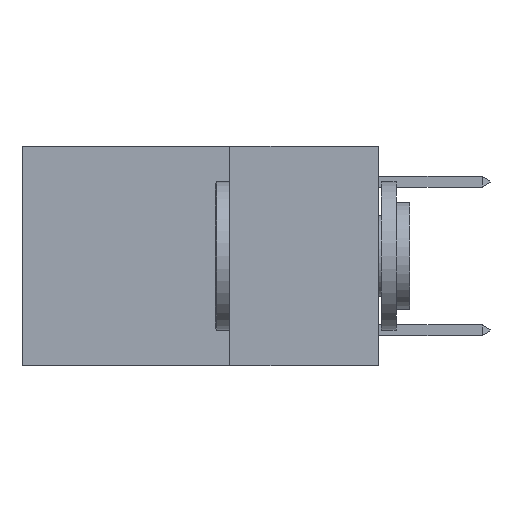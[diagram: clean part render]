
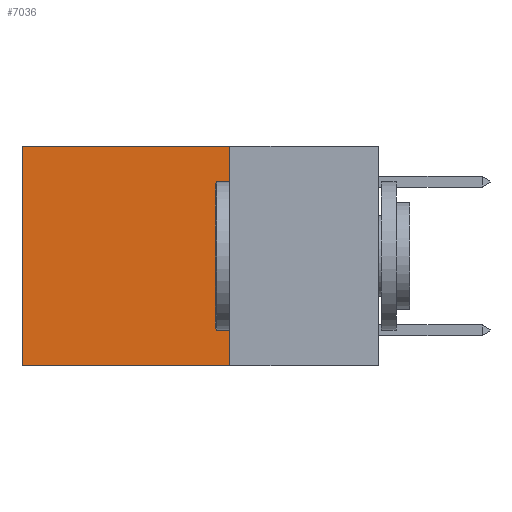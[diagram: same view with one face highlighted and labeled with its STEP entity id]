
A CAD part, left-side view. The second image highlights one B-rep face of the part: STEP entity #7036.
In plain terms, the highlighted planar face has unit normal (-1, 0, 0).
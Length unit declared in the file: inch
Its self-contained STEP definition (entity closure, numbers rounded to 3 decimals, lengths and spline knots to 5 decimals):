
#8 = AXIS2_PLACEMENT_3D ( 'NONE', #4700, #12351, #10849 ) ;
#154 = LINE ( 'NONE', #18532, #13078 ) ;
#290 = FACE_OUTER_BOUND ( 'NONE', #3960, .T. ) ;
#1508 = DIRECTION ( 'NONE',  ( 0., 0., -1. ) ) ;
#2467 = CARTESIAN_POINT ( 'NONE',  ( 0.2625, 0.25, -0.37 ) ) ;
#2901 = VECTOR ( 'NONE', #1508, 39.37008 ) ;
#2958 = VERTEX_POINT ( 'NONE', #6874 ) ;
#3917 = LINE ( 'NONE', #13137, #6605 ) ;
#3960 = EDGE_LOOP ( 'NONE', ( #4642, #15360, #17012, #11257 ) ) ;
#4370 = EDGE_CURVE ( 'NONE', #17530, #2958, #154, .T. ) ;
#4642 = ORIENTED_EDGE ( 'NONE', *, *, #4370, .T. ) ;
#4700 = CARTESIAN_POINT ( 'NONE',  ( 0.2625, 0.25, 0. ) ) ;
#4904 = PLANE ( 'NONE',  #8 ) ;
#5879 = DIRECTION ( 'NONE',  ( 0., 1., 0. ) ) ;
#6605 = VECTOR ( 'NONE', #17549, 39.37008 ) ;
#6691 = EDGE_CURVE ( 'NONE', #14628, #8498, #11177, .T. ) ;
#6874 = CARTESIAN_POINT ( 'NONE',  ( 0.2625, 0.6, -0.37 ) ) ;
#7036 = ADVANCED_FACE ( 'NONE', ( #290 ), #4904, .F. ) ;
#7203 = LINE ( 'NONE', #2467, #10703 ) ;
#7423 = CARTESIAN_POINT ( 'NONE',  ( 0.2625, 0.25, -0.37 ) ) ;
#8498 = VERTEX_POINT ( 'NONE', #7423 ) ;
#10481 = EDGE_CURVE ( 'NONE', #8498, #2958, #7203, .T. ) ;
#10703 = VECTOR ( 'NONE', #5879, 39.37008 ) ;
#10849 = DIRECTION ( 'NONE',  ( 0., 0., -1. ) ) ;
#11114 = CARTESIAN_POINT ( 'NONE',  ( 0.2625, 0.6, 0. ) ) ;
#11177 = LINE ( 'NONE', #15254, #2901 ) ;
#11257 = ORIENTED_EDGE ( 'NONE', *, *, #18497, .T. ) ;
#12351 = DIRECTION ( 'NONE',  ( 1., 0., 0. ) ) ;
#13078 = VECTOR ( 'NONE', #18635, 39.37008 ) ;
#13137 = CARTESIAN_POINT ( 'NONE',  ( 0.2625, 0.25, 0. ) ) ;
#14628 = VERTEX_POINT ( 'NONE', #19581 ) ;
#15254 = CARTESIAN_POINT ( 'NONE',  ( 0.2625, 0.25, 0. ) ) ;
#15360 = ORIENTED_EDGE ( 'NONE', *, *, #10481, .F. ) ;
#17012 = ORIENTED_EDGE ( 'NONE', *, *, #6691, .F. ) ;
#17530 = VERTEX_POINT ( 'NONE', #11114 ) ;
#17549 = DIRECTION ( 'NONE',  ( 0., 1., 0. ) ) ;
#18497 = EDGE_CURVE ( 'NONE', #14628, #17530, #3917, .T. ) ;
#18532 = CARTESIAN_POINT ( 'NONE',  ( 0.2625, 0.6, 0. ) ) ;
#18635 = DIRECTION ( 'NONE',  ( 0., 0., -1. ) ) ;
#19581 = CARTESIAN_POINT ( 'NONE',  ( 0.2625, 0.25, 0. ) ) ;
